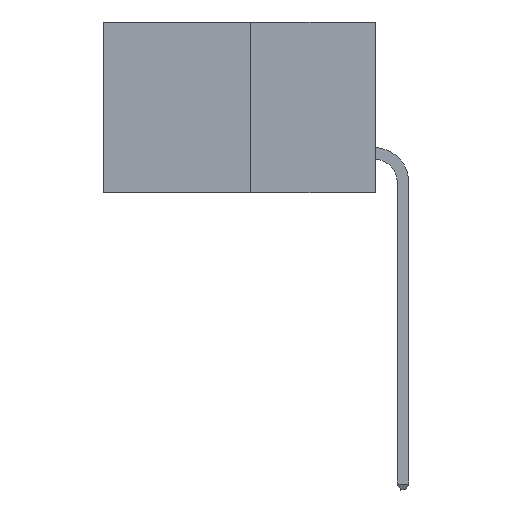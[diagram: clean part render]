
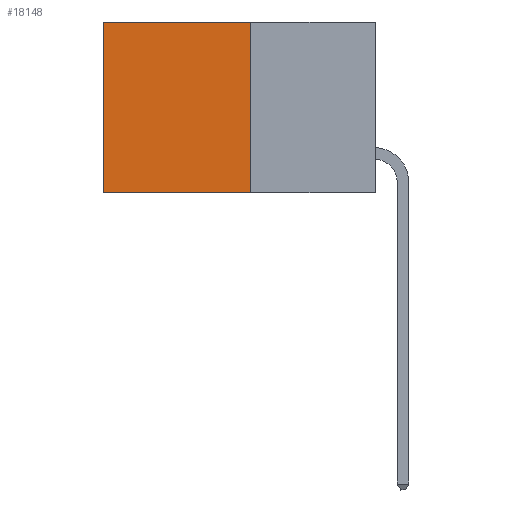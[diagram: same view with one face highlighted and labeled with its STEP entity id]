
A CAD part, left-side view. The second image highlights one B-rep face of the part: STEP entity #18148.
In plain terms, the highlighted planar face has unit normal (-1, 0, 0).
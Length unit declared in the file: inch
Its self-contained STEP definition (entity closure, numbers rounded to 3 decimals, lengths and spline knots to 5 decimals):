
#947 = VERTEX_POINT ( 'NONE', #26079 ) ;
#3042 = VECTOR ( 'NONE', #25629, 39.37008 ) ;
#3102 = ORIENTED_EDGE ( 'NONE', *, *, #22551, .F. ) ;
#3727 = ORIENTED_EDGE ( 'NONE', *, *, #22418, .T. ) ;
#4087 = ORIENTED_EDGE ( 'NONE', *, *, #22715, .F. ) ;
#4446 = DIRECTION ( 'NONE',  ( 0., 0., -1. ) ) ;
#5664 = CARTESIAN_POINT ( 'NONE',  ( 0.277, 0.27, -0.37 ) ) ;
#6418 = PLANE ( 'NONE',  #14132 ) ;
#6523 = LINE ( 'NONE', #5664, #16809 ) ;
#8101 = VERTEX_POINT ( 'NONE', #24457 ) ;
#8464 = DIRECTION ( 'NONE',  ( 0., 0., -1. ) ) ;
#8812 = VERTEX_POINT ( 'NONE', #22679 ) ;
#8960 = EDGE_CURVE ( 'NONE', #947, #8101, #19352, .T. ) ;
#9815 = VERTEX_POINT ( 'NONE', #26039 ) ;
#12449 = EDGE_LOOP ( 'NONE', ( #3727, #3102, #4087, #24675 ) ) ;
#14132 = AXIS2_PLACEMENT_3D ( 'NONE', #14587, #20776, #8464 ) ;
#14587 = CARTESIAN_POINT ( 'NONE',  ( 0.277, 0.27, -0.37 ) ) ;
#14620 = CARTESIAN_POINT ( 'NONE',  ( 0.277, 0.59, -0.37 ) ) ;
#15817 = LINE ( 'NONE', #19156, #20645 ) ;
#15837 = DIRECTION ( 'NONE',  ( 0., 0., -1. ) ) ;
#16809 = VECTOR ( 'NONE', #15837, 39.37008 ) ;
#18148 = ADVANCED_FACE ( 'NONE', ( #22692 ), #6418, .F. ) ;
#18406 = VECTOR ( 'NONE', #4446, 39.37008 ) ;
#19156 = CARTESIAN_POINT ( 'NONE',  ( 0.277, 0.27, -0.37 ) ) ;
#19352 = LINE ( 'NONE', #23607, #3042 ) ;
#20645 = VECTOR ( 'NONE', #21248, 39.37008 ) ;
#20776 = DIRECTION ( 'NONE',  ( 1., 0., 0. ) ) ;
#21248 = DIRECTION ( 'NONE',  ( 0., 1., 0. ) ) ;
#22418 = EDGE_CURVE ( 'NONE', #8101, #9815, #23856, .T. ) ;
#22551 = EDGE_CURVE ( 'NONE', #8812, #9815, #15817, .T. ) ;
#22679 = CARTESIAN_POINT ( 'NONE',  ( 0.277, 0.27, -0.37 ) ) ;
#22692 = FACE_OUTER_BOUND ( 'NONE', #12449, .T. ) ;
#22715 = EDGE_CURVE ( 'NONE', #947, #8812, #6523, .T. ) ;
#23607 = CARTESIAN_POINT ( 'NONE',  ( 0.277, 0.27, 0. ) ) ;
#23856 = LINE ( 'NONE', #14620, #18406 ) ;
#24457 = CARTESIAN_POINT ( 'NONE',  ( 0.277, 0.59, 0. ) ) ;
#24675 = ORIENTED_EDGE ( 'NONE', *, *, #8960, .T. ) ;
#25629 = DIRECTION ( 'NONE',  ( 0., 1., 0. ) ) ;
#26039 = CARTESIAN_POINT ( 'NONE',  ( 0.277, 0.59, -0.37 ) ) ;
#26079 = CARTESIAN_POINT ( 'NONE',  ( 0.277, 0.27, 0. ) ) ;
